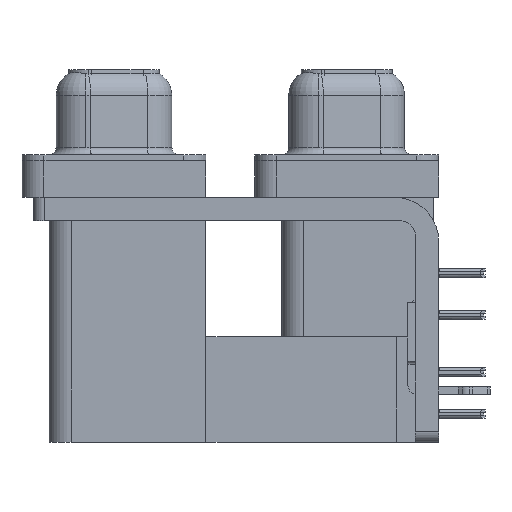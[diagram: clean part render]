
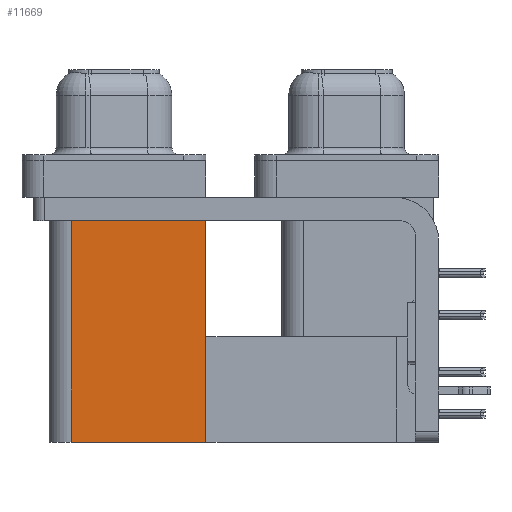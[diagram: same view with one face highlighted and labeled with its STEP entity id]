
A CAD part, left-side view. The second image highlights one B-rep face of the part: STEP entity #11669.
In plain terms, the highlighted planar face has unit normal (-1, 0, 0).
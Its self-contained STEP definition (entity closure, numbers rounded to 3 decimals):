
#2259 = CARTESIAN_POINT ( 'NONE',  ( 3.765, 9.6, -2.5 ) ) ;
#3988 = VERTEX_POINT ( 'NONE', #23353 ) ;
#5286 = ORIENTED_EDGE ( 'NONE', *, *, #27351, .T. ) ;
#6231 = DIRECTION ( 'NONE',  ( 1., 0., 0. ) ) ;
#6352 = EDGE_CURVE ( 'NONE', #22733, #3988, #49482, .T. ) ;
#7343 = EDGE_CURVE ( 'NONE', #42115, #35129, #18503, .T. ) ;
#8238 = EDGE_LOOP ( 'NONE', ( #11997, #35372, #16260, #5286 ) ) ;
#8775 = VECTOR ( 'NONE', #22328, 1000. ) ;
#10075 = FACE_OUTER_BOUND ( 'NONE', #8238, .T. ) ;
#10224 = DIRECTION ( 'NONE',  ( 0., 1., 0. ) ) ;
#11481 = AXIS2_PLACEMENT_3D ( 'NONE', #30068, #6231, #33407 ) ;
#11669 = ADVANCED_FACE ( 'NONE', ( #10075 ), #37508, .F. ) ;
#11872 = VECTOR ( 'NONE', #30625, 1000. ) ;
#11997 = ORIENTED_EDGE ( 'NONE', *, *, #6352, .T. ) ;
#13981 = CARTESIAN_POINT ( 'NONE',  ( 3.765, 9.6, -19.2 ) ) ;
#16260 = ORIENTED_EDGE ( 'NONE', *, *, #7343, .F. ) ;
#18503 = LINE ( 'NONE', #26187, #8775 ) ;
#19597 = VECTOR ( 'NONE', #32973, 1000. ) ;
#21704 = CARTESIAN_POINT ( 'NONE',  ( 3.765, 18.8, -19.2 ) ) ;
#22328 = DIRECTION ( 'NONE',  ( 0., 1., 0. ) ) ;
#22733 = VERTEX_POINT ( 'NONE', #50439 ) ;
#23353 = CARTESIAN_POINT ( 'NONE',  ( 3.765, 18.8, -2.5 ) ) ;
#23388 = VECTOR ( 'NONE', #10224, 1000. ) ;
#26187 = CARTESIAN_POINT ( 'NONE',  ( 3.765, 9.6, -19.2 ) ) ;
#27351 = EDGE_CURVE ( 'NONE', #42115, #22733, #30129, .T. ) ;
#30068 = CARTESIAN_POINT ( 'NONE',  ( 3.765, 9.6, -19.2 ) ) ;
#30129 = LINE ( 'NONE', #45791, #11872 ) ;
#30625 = DIRECTION ( 'NONE',  ( 0., 0., 1. ) ) ;
#32973 = DIRECTION ( 'NONE',  ( 0., 0., 1. ) ) ;
#33407 = DIRECTION ( 'NONE',  ( 0., 0., -1. ) ) ;
#35129 = VERTEX_POINT ( 'NONE', #38401 ) ;
#35299 = EDGE_CURVE ( 'NONE', #35129, #3988, #41192, .T. ) ;
#35372 = ORIENTED_EDGE ( 'NONE', *, *, #35299, .F. ) ;
#37508 = PLANE ( 'NONE',  #11481 ) ;
#38401 = CARTESIAN_POINT ( 'NONE',  ( 3.765, 18.8, -19.2 ) ) ;
#41192 = LINE ( 'NONE', #21704, #19597 ) ;
#42115 = VERTEX_POINT ( 'NONE', #13981 ) ;
#45791 = CARTESIAN_POINT ( 'NONE',  ( 3.765, 9.6, -19.2 ) ) ;
#49482 = LINE ( 'NONE', #2259, #23388 ) ;
#50439 = CARTESIAN_POINT ( 'NONE',  ( 3.765, 9.6, -2.5 ) ) ;
